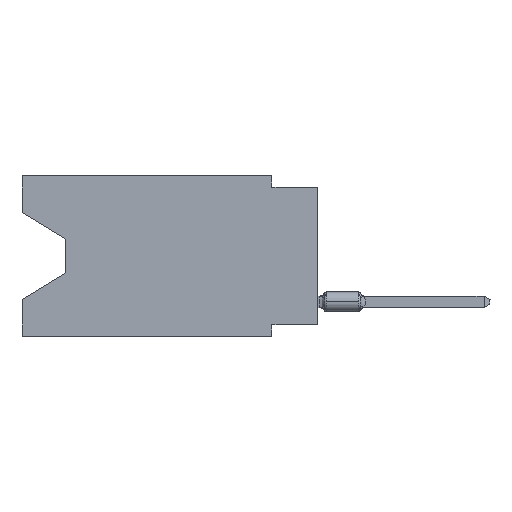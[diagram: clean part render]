
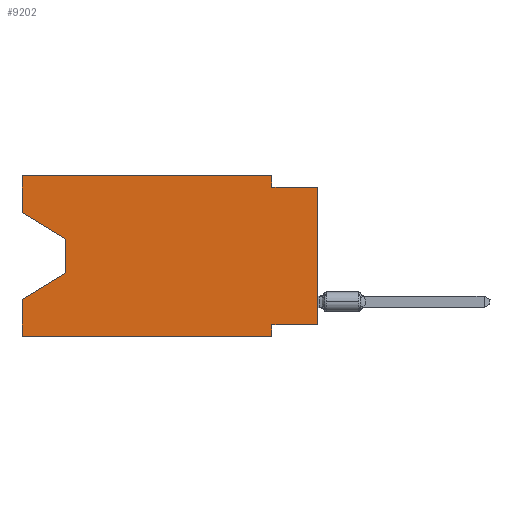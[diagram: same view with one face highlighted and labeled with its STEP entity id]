
A CAD part, left-side view. The second image highlights one B-rep face of the part: STEP entity #9202.
In plain terms, the highlighted planar face has unit normal (-1, 0, 0).
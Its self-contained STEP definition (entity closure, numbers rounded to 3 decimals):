
#154 = ORIENTED_EDGE ( 'NONE', *, *, #34295, .T. ) ;
#223 = LINE ( 'NONE', #47191, #38032 ) ;
#358 = DIRECTION ( 'NONE',  ( 0., 1., 0. ) ) ;
#1140 = ORIENTED_EDGE ( 'NONE', *, *, #39042, .F. ) ;
#1400 = LINE ( 'NONE', #39822, #47535 ) ;
#1483 = CARTESIAN_POINT ( 'NONE',  ( 0., 2.54, -0.635 ) ) ;
#2694 = LINE ( 'NONE', #10945, #40215 ) ;
#2915 = LINE ( 'NONE', #22234, #42003 ) ;
#3242 = DIRECTION ( 'NONE',  ( 0., -0.855, -0.519 ) ) ;
#4375 = DIRECTION ( 'NONE',  ( 0., 0., 1. ) ) ;
#4870 = CARTESIAN_POINT ( 'NONE',  ( 0., 0., -8.255 ) ) ;
#4955 = ORIENTED_EDGE ( 'NONE', *, *, #15739, .T. ) ;
#5044 = VECTOR ( 'NONE', #36855, 1000. ) ;
#5536 = DIRECTION ( 'NONE',  ( 1., 0., 0. ) ) ;
#5936 = CARTESIAN_POINT ( 'NONE',  ( 0., 2.54, -8.89 ) ) ;
#6461 = CARTESIAN_POINT ( 'NONE',  ( 0., 0., -0.635 ) ) ;
#6497 = CARTESIAN_POINT ( 'NONE',  ( 0., 13.97, -5.385 ) ) ;
#6944 = DIRECTION ( 'NONE',  ( 0., 0., 1. ) ) ;
#7381 = VERTEX_POINT ( 'NONE', #42499 ) ;
#7534 = CARTESIAN_POINT ( 'NONE',  ( 0., 16.383, -8.89 ) ) ;
#8504 = VECTOR ( 'NONE', #9347, 1000. ) ;
#9202 = ADVANCED_FACE ( 'NONE', ( #24611 ), #48489, .F. ) ;
#9347 = DIRECTION ( 'NONE',  ( 0., 0., -1. ) ) ;
#9386 = EDGE_CURVE ( 'NONE', #28906, #21432, #223, .T. ) ;
#9898 = ORIENTED_EDGE ( 'NONE', *, *, #46351, .F. ) ;
#10484 = CARTESIAN_POINT ( 'NONE',  ( 0., 13.97, -3.505 ) ) ;
#10945 = CARTESIAN_POINT ( 'NONE',  ( 0., 0., 0. ) ) ;
#12128 = VERTEX_POINT ( 'NONE', #1483 ) ;
#12191 = ORIENTED_EDGE ( 'NONE', *, *, #9386, .T. ) ;
#12596 = VERTEX_POINT ( 'NONE', #27560 ) ;
#13437 = CARTESIAN_POINT ( 'NONE',  ( 0., 13.97, -5.385 ) ) ;
#13795 = ORIENTED_EDGE ( 'NONE', *, *, #48727, .F. ) ;
#14844 = CARTESIAN_POINT ( 'NONE',  ( 0., 0., -0.635 ) ) ;
#15739 = EDGE_CURVE ( 'NONE', #29818, #25591, #2694, .T. ) ;
#15872 = LINE ( 'NONE', #20416, #8504 ) ;
#15886 = LINE ( 'NONE', #4870, #40330 ) ;
#16142 = LINE ( 'NONE', #27727, #29090 ) ;
#18708 = EDGE_LOOP ( 'NONE', ( #32132, #154, #41704, #13795, #12191, #1140, #36906, #4955, #22235, #9898, #26122, #31536 ) ) ;
#19253 = CARTESIAN_POINT ( 'NONE',  ( 0., 16.383, -2.038 ) ) ;
#19333 = VECTOR ( 'NONE', #40426, 1000. ) ;
#20416 = CARTESIAN_POINT ( 'NONE',  ( 0., 2.54, 0. ) ) ;
#21432 = VERTEX_POINT ( 'NONE', #49051 ) ;
#21798 = LINE ( 'NONE', #10484, #37603 ) ;
#22144 = CARTESIAN_POINT ( 'NONE',  ( 0., 2.54, -8.255 ) ) ;
#22234 = CARTESIAN_POINT ( 'NONE',  ( 0., 16.383, 0. ) ) ;
#22235 = ORIENTED_EDGE ( 'NONE', *, *, #42382, .F. ) ;
#24611 = FACE_OUTER_BOUND ( 'NONE', #18708, .T. ) ;
#25402 = CARTESIAN_POINT ( 'NONE',  ( 0., 16.383, -2.038 ) ) ;
#25591 = VERTEX_POINT ( 'NONE', #14844 ) ;
#25631 = VERTEX_POINT ( 'NONE', #22144 ) ;
#26071 = EDGE_CURVE ( 'NONE', #49201, #12596, #16142, .T. ) ;
#26122 = ORIENTED_EDGE ( 'NONE', *, *, #42590, .F. ) ;
#27560 = CARTESIAN_POINT ( 'NONE',  ( 0., 16.383, 0. ) ) ;
#27727 = CARTESIAN_POINT ( 'NONE',  ( 0., 16.383, 0. ) ) ;
#28640 = CARTESIAN_POINT ( 'NONE',  ( 0., 16.383, 0. ) ) ;
#28906 = VERTEX_POINT ( 'NONE', #7534 ) ;
#29069 = DIRECTION ( 'NONE',  ( 0., 0., 1. ) ) ;
#29090 = VECTOR ( 'NONE', #4375, 1000. ) ;
#29114 = LINE ( 'NONE', #6497, #19333 ) ;
#29818 = VERTEX_POINT ( 'NONE', #49626 ) ;
#30682 = CARTESIAN_POINT ( 'NONE',  ( 0., 2.54, 0. ) ) ;
#31351 = VECTOR ( 'NONE', #39344, 1000. ) ;
#31536 = ORIENTED_EDGE ( 'NONE', *, *, #26071, .F. ) ;
#32132 = ORIENTED_EDGE ( 'NONE', *, *, #39890, .T. ) ;
#34295 = EDGE_CURVE ( 'NONE', #47060, #37911, #21798, .T. ) ;
#35575 = AXIS2_PLACEMENT_3D ( 'NONE', #28640, #5536, #40926 ) ;
#35584 = EDGE_CURVE ( 'NONE', #37911, #7381, #29114, .T. ) ;
#36855 = DIRECTION ( 'NONE',  ( 0., -1., 0. ) ) ;
#36898 = VERTEX_POINT ( 'NONE', #30682 ) ;
#36906 = ORIENTED_EDGE ( 'NONE', *, *, #40876, .F. ) ;
#37603 = VECTOR ( 'NONE', #40160, 1000. ) ;
#37911 = VERTEX_POINT ( 'NONE', #13437 ) ;
#38032 = VECTOR ( 'NONE', #46700, 1000. ) ;
#38585 = CARTESIAN_POINT ( 'NONE',  ( 0., 13.97, -3.505 ) ) ;
#38839 = DIRECTION ( 'NONE',  ( 0., -1., 0. ) ) ;
#39042 = EDGE_CURVE ( 'NONE', #25631, #21432, #44122, .T. ) ;
#39344 = DIRECTION ( 'NONE',  ( 0., 0., -1. ) ) ;
#39458 = VECTOR ( 'NONE', #3242, 1000. ) ;
#39822 = CARTESIAN_POINT ( 'NONE',  ( 0., 16.383, 0. ) ) ;
#39890 = EDGE_CURVE ( 'NONE', #49201, #47060, #45687, .T. ) ;
#40160 = DIRECTION ( 'NONE',  ( 0., 0., -1. ) ) ;
#40215 = VECTOR ( 'NONE', #6944, 1000. ) ;
#40330 = VECTOR ( 'NONE', #358, 1000. ) ;
#40426 = DIRECTION ( 'NONE',  ( 0., 0.855, -0.519 ) ) ;
#40865 = LINE ( 'NONE', #6461, #5044 ) ;
#40876 = EDGE_CURVE ( 'NONE', #29818, #25631, #15886, .T. ) ;
#40926 = DIRECTION ( 'NONE',  ( 0., 0., -1. ) ) ;
#41704 = ORIENTED_EDGE ( 'NONE', *, *, #35584, .T. ) ;
#42003 = VECTOR ( 'NONE', #29069, 1000. ) ;
#42382 = EDGE_CURVE ( 'NONE', #12128, #25591, #40865, .T. ) ;
#42499 = CARTESIAN_POINT ( 'NONE',  ( 0., 16.383, -6.852 ) ) ;
#42590 = EDGE_CURVE ( 'NONE', #12596, #36898, #1400, .T. ) ;
#44122 = LINE ( 'NONE', #5936, #31351 ) ;
#45687 = LINE ( 'NONE', #25402, #39458 ) ;
#46351 = EDGE_CURVE ( 'NONE', #36898, #12128, #15872, .T. ) ;
#46700 = DIRECTION ( 'NONE',  ( 0., -1., 0. ) ) ;
#47060 = VERTEX_POINT ( 'NONE', #38585 ) ;
#47191 = CARTESIAN_POINT ( 'NONE',  ( 0., 16.383, -8.89 ) ) ;
#47535 = VECTOR ( 'NONE', #38839, 1000. ) ;
#48489 = PLANE ( 'NONE',  #35575 ) ;
#48727 = EDGE_CURVE ( 'NONE', #28906, #7381, #2915, .T. ) ;
#49051 = CARTESIAN_POINT ( 'NONE',  ( 0., 2.54, -8.89 ) ) ;
#49201 = VERTEX_POINT ( 'NONE', #19253 ) ;
#49626 = CARTESIAN_POINT ( 'NONE',  ( 0., 0., -8.255 ) ) ;
